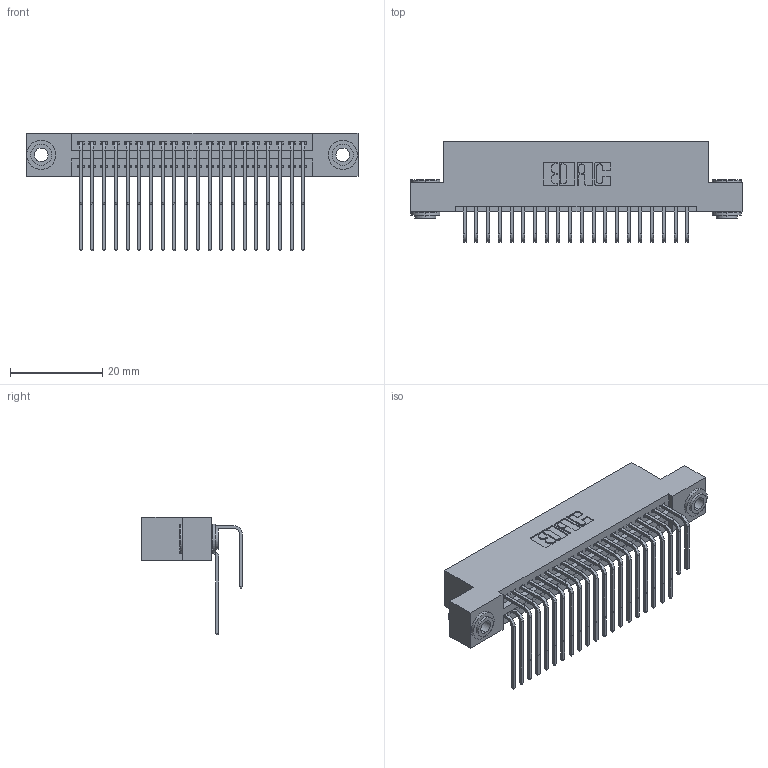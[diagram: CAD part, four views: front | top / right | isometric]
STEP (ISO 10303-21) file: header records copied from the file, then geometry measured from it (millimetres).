
FILE_DESCRIPTION (( 'STEP AP203' ), '1' );
FILE_NAME ('345-040-558-203.STEP', '2019-10-28T18:25:58', ( '' ), ( '' ), 'SwSTEP 2.0', 'SolidWorks 2016', '' );
FILE_SCHEMA (( 'CONFIG_CONTROL_DESIGN' ));
Length unit declared in the file: inch
Products named in the file (5): 345 Part_Flush Mounting Lugs - 0.156 Dia-TH; 345-292-001_558 Tail - 2; 345-040-558-203; 345-250-002_345-250-002-102; 345-292-001_558 559 Tail - 1
Assembly tree (43 placements, depth 2):
  345-040-558-203
    345 Part_Flush Mounting Lugs - 0.156 Dia-TH
    345-292-001_558 559 Tail - 1  x20
    345-292-001_558 Tail - 2  x20
    345-250-002_345-250-002-102  x2
Bounding box: 72.01 x 21.83 x 25.53 mm (x, y, z)
Volume: 7041 mm3; surface area: 11271.6 mm2
Topology: 43 solids, 43 shells, 2244 faces, 6617 edges, 4354 vertices
Faces by surface type: plane 1490, cylinder 746, cone 8
Entity records: 20956 total; most frequent: CARTESIAN_POINT 3554, ORIENTED_EDGE 3430, DIRECTION 3165, EDGE_CURVE 1715, VECTOR 1439, LINE 1439, VERTEX_POINT 1138, AXIS2_PLACEMENT_3D 863
